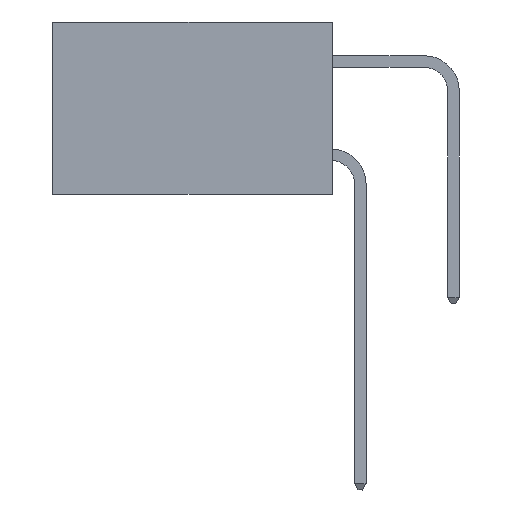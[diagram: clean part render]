
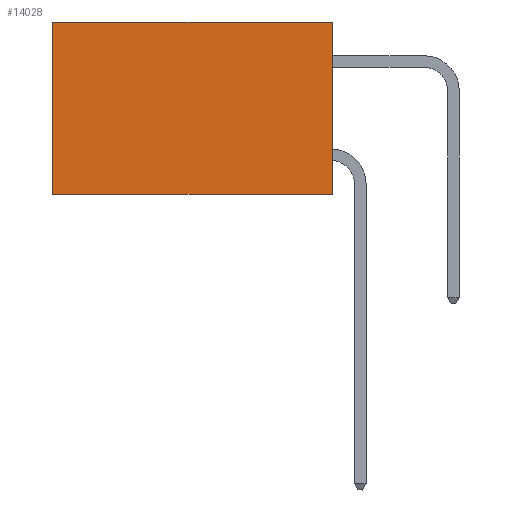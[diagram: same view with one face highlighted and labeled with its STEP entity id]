
A CAD part, left-side view. The second image highlights one B-rep face of the part: STEP entity #14028.
In plain terms, the highlighted planar face has unit normal (-1, 0, 0).
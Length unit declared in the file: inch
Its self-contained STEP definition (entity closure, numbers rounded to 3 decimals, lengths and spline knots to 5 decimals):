
#315 = CARTESIAN_POINT ( 'NONE',  ( 0.298, 0., 0. ) ) ;
#799 = DIRECTION ( 'NONE',  ( 0., 1., 0. ) ) ;
#1011 = CARTESIAN_POINT ( 'NONE',  ( 0.298, 0., -0.37 ) ) ;
#1915 = CARTESIAN_POINT ( 'NONE',  ( 0.298, 0.6, 0. ) ) ;
#3163 = DIRECTION ( 'NONE',  ( 0., 1., 0. ) ) ;
#3812 = VERTEX_POINT ( 'NONE', #23261 ) ;
#4549 = DIRECTION ( 'NONE',  ( 0., 0., -1. ) ) ;
#5138 = DIRECTION ( 'NONE',  ( 0., 0., -1. ) ) ;
#5197 = LINE ( 'NONE', #23739, #11527 ) ;
#6498 = VERTEX_POINT ( 'NONE', #1915 ) ;
#6720 = DIRECTION ( 'NONE',  ( 1., 0., 0. ) ) ;
#7688 = PLANE ( 'NONE',  #19868 ) ;
#8126 = VERTEX_POINT ( 'NONE', #16961 ) ;
#9537 = DIRECTION ( 'NONE',  ( 0., 0., -1. ) ) ;
#11362 = ORIENTED_EDGE ( 'NONE', *, *, #21964, .F. ) ;
#11364 = ORIENTED_EDGE ( 'NONE', *, *, #25018, .T. ) ;
#11527 = VECTOR ( 'NONE', #799, 39.37008 ) ;
#11695 = VECTOR ( 'NONE', #3163, 39.37008 ) ;
#12360 = LINE ( 'NONE', #1011, #11695 ) ;
#13152 = ORIENTED_EDGE ( 'NONE', *, *, #18412, .F. ) ;
#14028 = ADVANCED_FACE ( 'NONE', ( #20696 ), #7688, .F. ) ;
#16730 = VERTEX_POINT ( 'NONE', #20559 ) ;
#16961 = CARTESIAN_POINT ( 'NONE',  ( 0.298, 0.6, -0.37 ) ) ;
#18233 = CARTESIAN_POINT ( 'NONE',  ( 0.298, 0.6, 0. ) ) ;
#18412 = EDGE_CURVE ( 'NONE', #3812, #8126, #12360, .T. ) ;
#18502 = EDGE_LOOP ( 'NONE', ( #11364, #13152, #11362, #24505 ) ) ;
#19868 = AXIS2_PLACEMENT_3D ( 'NONE', #315, #6720, #4549 ) ;
#20140 = CARTESIAN_POINT ( 'NONE',  ( 0.298, 0., 0. ) ) ;
#20559 = CARTESIAN_POINT ( 'NONE',  ( 0.298, 0., 0. ) ) ;
#20677 = VECTOR ( 'NONE', #5138, 39.37008 ) ;
#20696 = FACE_OUTER_BOUND ( 'NONE', #18502, .T. ) ;
#21809 = VECTOR ( 'NONE', #9537, 39.37008 ) ;
#21964 = EDGE_CURVE ( 'NONE', #16730, #3812, #24471, .T. ) ;
#22407 = EDGE_CURVE ( 'NONE', #16730, #6498, #5197, .T. ) ;
#23261 = CARTESIAN_POINT ( 'NONE',  ( 0.298, 0., -0.37 ) ) ;
#23739 = CARTESIAN_POINT ( 'NONE',  ( 0.298, 0., 0. ) ) ;
#24471 = LINE ( 'NONE', #20140, #21809 ) ;
#24505 = ORIENTED_EDGE ( 'NONE', *, *, #22407, .T. ) ;
#25018 = EDGE_CURVE ( 'NONE', #6498, #8126, #27344, .T. ) ;
#27344 = LINE ( 'NONE', #18233, #20677 ) ;
